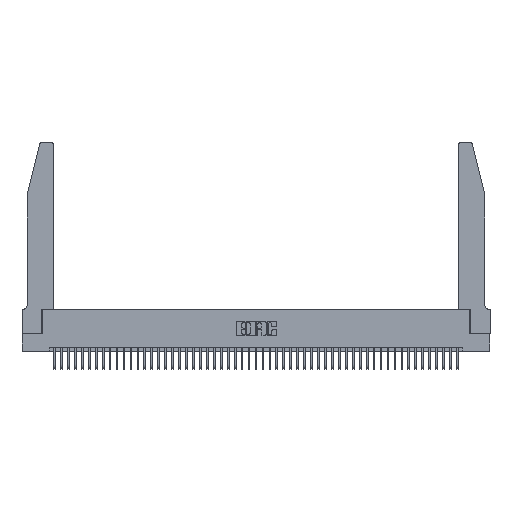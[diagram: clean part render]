
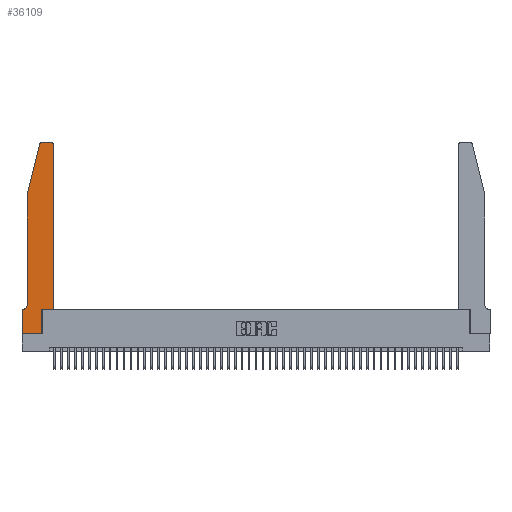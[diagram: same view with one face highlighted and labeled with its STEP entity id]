
A CAD part, top view. The second image highlights one B-rep face of the part: STEP entity #36109.
In plain terms, the highlighted planar face has unit normal (0, 0, 1).
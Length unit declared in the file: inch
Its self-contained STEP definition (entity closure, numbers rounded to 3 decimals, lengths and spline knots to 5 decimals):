
#383 = CARTESIAN_POINT ( 'NONE',  ( 0.0755, 2., 0.37 ) ) ;
#414 = LINE ( 'NONE', #24184, #43103 ) ;
#569 = CARTESIAN_POINT ( 'NONE',  ( 0., 0., 0.37 ) ) ;
#829 = VERTEX_POINT ( 'NONE', #46330 ) ;
#1275 = PLANE ( 'NONE',  #25282 ) ;
#2001 = CARTESIAN_POINT ( 'NONE',  ( 0.2865, 0.35, 0.37 ) ) ;
#2657 = DIRECTION ( 'NONE',  ( -0.239, -0.971, 0. ) ) ;
#3106 = EDGE_CURVE ( 'NONE', #22132, #20932, #33323, .T. ) ;
#3316 = VECTOR ( 'NONE', #11721, 39.37008 ) ;
#4582 = DIRECTION ( 'NONE',  ( 0., 0., 1. ) ) ;
#4771 = CARTESIAN_POINT ( 'NONE',  ( 0.0755, 0.35, 0.37 ) ) ;
#5614 = VECTOR ( 'NONE', #32003, 39.37008 ) ;
#6603 = DIRECTION ( 'NONE',  ( 0., -1., 0. ) ) ;
#6908 = LINE ( 'NONE', #41653, #47162 ) ;
#7243 = CIRCLE ( 'NONE', #15041, 0.07 ) ;
#7301 = ORIENTED_EDGE ( 'NONE', *, *, #30319, .T. ) ;
#7585 = CARTESIAN_POINT ( 'NONE',  ( 0.2865, 0.35, 0.37 ) ) ;
#7694 = CARTESIAN_POINT ( 'NONE',  ( 0., 0., 0.37 ) ) ;
#9131 = DIRECTION ( 'NONE',  ( 0., 0., 1. ) ) ;
#10009 = VERTEX_POINT ( 'NONE', #46419 ) ;
#10342 = CARTESIAN_POINT ( 'NONE',  ( 0.0755, 2., 0.37 ) ) ;
#10405 = DIRECTION ( 'NONE',  ( 0., 0., -1. ) ) ;
#11170 = EDGE_CURVE ( 'NONE', #24450, #48132, #28840, .T. ) ;
#11181 = EDGE_CURVE ( 'NONE', #38660, #24450, #6908, .T. ) ;
#11345 = ORIENTED_EDGE ( 'NONE', *, *, #30544, .T. ) ;
#11398 = ORIENTED_EDGE ( 'NONE', *, *, #45949, .T. ) ;
#11414 = AXIS2_PLACEMENT_3D ( 'NONE', #27939, #4582, #31828 ) ;
#11721 = DIRECTION ( 'NONE',  ( 0., 1., 0. ) ) ;
#13100 = CARTESIAN_POINT ( 'NONE',  ( 0.4205, 2.72, 0.37 ) ) ;
#13160 = CARTESIAN_POINT ( 'NONE',  ( 0., 0., 0.37 ) ) ;
#13324 = DIRECTION ( 'NONE',  ( 0., -1., 0. ) ) ;
#13718 = LINE ( 'NONE', #31114, #3316 ) ;
#13916 = ORIENTED_EDGE ( 'NONE', *, *, #11170, .T. ) ;
#14481 = EDGE_CURVE ( 'NONE', #34464, #829, #18198, .T. ) ;
#15041 = AXIS2_PLACEMENT_3D ( 'NONE', #33744, #10405, #37604 ) ;
#15719 = EDGE_CURVE ( 'NONE', #829, #46100, #42099, .T. ) ;
#17038 = DIRECTION ( 'NONE',  ( 1., 0., 0. ) ) ;
#17658 = VERTEX_POINT ( 'NONE', #7694 ) ;
#18198 = CIRCLE ( 'NONE', #32183, 0.03 ) ;
#18864 = ORIENTED_EDGE ( 'NONE', *, *, #3106, .T. ) ;
#19570 = ORIENTED_EDGE ( 'NONE', *, *, #42383, .T. ) ;
#19920 = ORIENTED_EDGE ( 'NONE', *, *, #47863, .T. ) ;
#20932 = VERTEX_POINT ( 'NONE', #2001 ) ;
#20966 = CARTESIAN_POINT ( 'NONE',  ( 0.2605, 2.75, 0.37 ) ) ;
#21751 = VECTOR ( 'NONE', #27011, 39.37008 ) ;
#22132 = VERTEX_POINT ( 'NONE', #40195 ) ;
#23236 = EDGE_CURVE ( 'NONE', #41913, #17658, #26342, .T. ) ;
#23286 = FACE_OUTER_BOUND ( 'NONE', #36342, .T. ) ;
#24184 = CARTESIAN_POINT ( 'NONE',  ( 0.4505, 0.35, 0.37 ) ) ;
#24381 = ORIENTED_EDGE ( 'NONE', *, *, #15719, .T. ) ;
#24423 = ORIENTED_EDGE ( 'NONE', *, *, #23236, .T. ) ;
#24450 = VERTEX_POINT ( 'NONE', #383 ) ;
#24748 = ORIENTED_EDGE ( 'NONE', *, *, #14481, .T. ) ;
#25113 = VECTOR ( 'NONE', #13324, 39.37008 ) ;
#25282 = AXIS2_PLACEMENT_3D ( 'NONE', #32449, #9131, #36354 ) ;
#26342 = LINE ( 'NONE', #13160, #25113 ) ;
#27011 = DIRECTION ( 'NONE',  ( 0., 1., 0. ) ) ;
#27939 = CARTESIAN_POINT ( 'NONE',  ( 0.284, 2.72, 0.37 ) ) ;
#28798 = LINE ( 'NONE', #569, #48301 ) ;
#28840 = LINE ( 'NONE', #10342, #36728 ) ;
#30319 = EDGE_CURVE ( 'NONE', #48132, #48631, #7243, .T. ) ;
#30517 = VECTOR ( 'NONE', #40338, 39.37008 ) ;
#30544 = EDGE_CURVE ( 'NONE', #46100, #38660, #46849, .T. ) ;
#31114 = CARTESIAN_POINT ( 'NONE',  ( 0.4505, 0.35, 0.37 ) ) ;
#31745 = DIRECTION ( 'NONE',  ( 1., 0., 0. ) ) ;
#31828 = DIRECTION ( 'NONE',  ( 1., 0., 0. ) ) ;
#31978 = DIRECTION ( 'NONE',  ( 1., 0., 0. ) ) ;
#32003 = DIRECTION ( 'NONE',  ( -1., 0., 0. ) ) ;
#32183 = AXIS2_PLACEMENT_3D ( 'NONE', #13100, #40271, #17038 ) ;
#32449 = CARTESIAN_POINT ( 'NONE',  ( 0., 0.35, 0.37 ) ) ;
#33323 = LINE ( 'NONE', #7585, #21751 ) ;
#33427 = CARTESIAN_POINT ( 'NONE',  ( 0.0755, 0.42, 0.37 ) ) ;
#33744 = CARTESIAN_POINT ( 'NONE',  ( 0.0055, 0.42, 0.37 ) ) ;
#34464 = VERTEX_POINT ( 'NONE', #36577 ) ;
#36109 = ADVANCED_FACE ( 'NONE', ( #23286 ), #1275, .T. ) ;
#36342 = EDGE_LOOP ( 'NONE', ( #24381, #11345, #45320, #13916, #7301, #11398, #24423, #19920, #18864, #19570, #46461, #24748 ) ) ;
#36354 = DIRECTION ( 'NONE',  ( 1., 0., 0. ) ) ;
#36577 = CARTESIAN_POINT ( 'NONE',  ( 0.4505, 2.72, 0.37 ) ) ;
#36728 = VECTOR ( 'NONE', #6603, 39.37008 ) ;
#37252 = CARTESIAN_POINT ( 'NONE',  ( 0., 0.35, 0.37 ) ) ;
#37604 = DIRECTION ( 'NONE',  ( -1., 0., 0. ) ) ;
#38660 = VERTEX_POINT ( 'NONE', #40269 ) ;
#40195 = CARTESIAN_POINT ( 'NONE',  ( 0.2865, 0., 0.37 ) ) ;
#40269 = CARTESIAN_POINT ( 'NONE',  ( 0.25487, 2.72718, 0.37 ) ) ;
#40271 = DIRECTION ( 'NONE',  ( 0., 0., 1. ) ) ;
#40338 = DIRECTION ( 'NONE',  ( -1., 0., 0. ) ) ;
#41653 = CARTESIAN_POINT ( 'NONE',  ( 0.0755, 2., 0.37 ) ) ;
#41913 = VERTEX_POINT ( 'NONE', #37252 ) ;
#42099 = LINE ( 'NONE', #20966, #30517 ) ;
#42383 = EDGE_CURVE ( 'NONE', #20932, #10009, #414, .T. ) ;
#43103 = VECTOR ( 'NONE', #31978, 39.37008 ) ;
#44586 = EDGE_CURVE ( 'NONE', #10009, #34464, #13718, .T. ) ;
#44625 = CARTESIAN_POINT ( 'NONE',  ( 0.284, 2.75, 0.37 ) ) ;
#44649 = CARTESIAN_POINT ( 'NONE',  ( 0.0055, 0.35, 0.37 ) ) ;
#45320 = ORIENTED_EDGE ( 'NONE', *, *, #11181, .T. ) ;
#45879 = LINE ( 'NONE', #4771, #5614 ) ;
#45949 = EDGE_CURVE ( 'NONE', #48631, #41913, #45879, .T. ) ;
#46100 = VERTEX_POINT ( 'NONE', #44625 ) ;
#46330 = CARTESIAN_POINT ( 'NONE',  ( 0.4205, 2.75, 0.37 ) ) ;
#46419 = CARTESIAN_POINT ( 'NONE',  ( 0.4505, 0.35, 0.37 ) ) ;
#46461 = ORIENTED_EDGE ( 'NONE', *, *, #44586, .T. ) ;
#46849 = CIRCLE ( 'NONE', #11414, 0.03 ) ;
#47162 = VECTOR ( 'NONE', #2657, 39.37008 ) ;
#47863 = EDGE_CURVE ( 'NONE', #17658, #22132, #28798, .T. ) ;
#48132 = VERTEX_POINT ( 'NONE', #33427 ) ;
#48301 = VECTOR ( 'NONE', #31745, 39.37008 ) ;
#48631 = VERTEX_POINT ( 'NONE', #44649 ) ;
